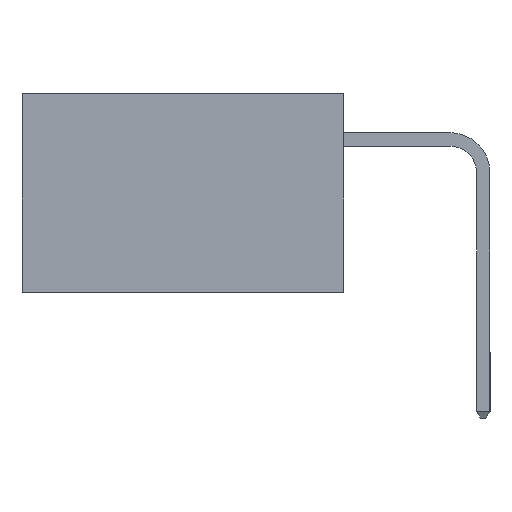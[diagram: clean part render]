
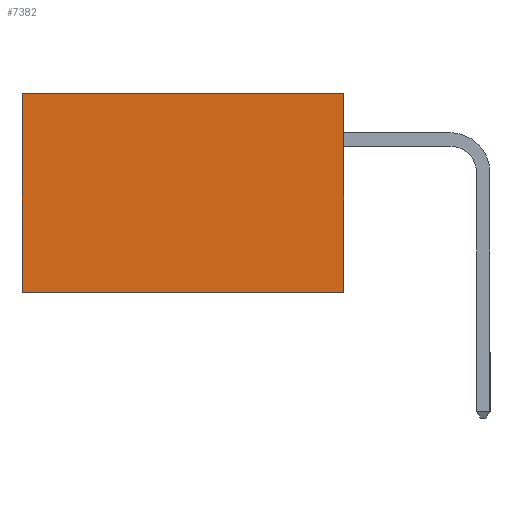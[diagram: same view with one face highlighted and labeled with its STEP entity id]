
A CAD part, left-side view. The second image highlights one B-rep face of the part: STEP entity #7382.
In plain terms, the highlighted planar face has unit normal (-1, 0, 0).
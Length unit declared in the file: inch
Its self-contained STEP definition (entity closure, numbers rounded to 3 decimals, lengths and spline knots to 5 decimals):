
#791 = CARTESIAN_POINT ( 'NONE',  ( 0.298, 0.6, 0. ) ) ;
#913 = VECTOR ( 'NONE', #17034, 39.37008 ) ;
#2879 = DIRECTION ( 'NONE',  ( 0., 1., 0. ) ) ;
#2944 = LINE ( 'NONE', #13796, #9721 ) ;
#3305 = ORIENTED_EDGE ( 'NONE', *, *, #6880, .F. ) ;
#4120 = CARTESIAN_POINT ( 'NONE',  ( 0.298, 0.6, -0.37 ) ) ;
#4395 = EDGE_CURVE ( 'NONE', #13428, #15532, #15515, .T. ) ;
#5298 = CARTESIAN_POINT ( 'NONE',  ( 0.298, 0., -0.37 ) ) ;
#5395 = VERTEX_POINT ( 'NONE', #5298 ) ;
#5860 = LINE ( 'NONE', #5873, #13768 ) ;
#5873 = CARTESIAN_POINT ( 'NONE',  ( 0.298, 0., -0.37 ) ) ;
#5914 = FACE_OUTER_BOUND ( 'NONE', #11638, .T. ) ;
#6100 = DIRECTION ( 'NONE',  ( 0., 0., -1. ) ) ;
#6880 = EDGE_CURVE ( 'NONE', #13428, #5395, #2944, .T. ) ;
#7157 = ORIENTED_EDGE ( 'NONE', *, *, #10382, .T. ) ;
#7382 = ADVANCED_FACE ( 'NONE', ( #5914 ), #11649, .F. ) ;
#7523 = DIRECTION ( 'NONE',  ( 1., 0., 0. ) ) ;
#8343 = LINE ( 'NONE', #17025, #13786 ) ;
#8783 = VERTEX_POINT ( 'NONE', #4120 ) ;
#9721 = VECTOR ( 'NONE', #13739, 39.37008 ) ;
#10382 = EDGE_CURVE ( 'NONE', #15532, #8783, #8343, .T. ) ;
#10694 = AXIS2_PLACEMENT_3D ( 'NONE', #11542, #7523, #15644 ) ;
#11014 = ORIENTED_EDGE ( 'NONE', *, *, #11450, .F. ) ;
#11450 = EDGE_CURVE ( 'NONE', #5395, #8783, #5860, .T. ) ;
#11542 = CARTESIAN_POINT ( 'NONE',  ( 0.298, 0., 0. ) ) ;
#11638 = EDGE_LOOP ( 'NONE', ( #7157, #11014, #3305, #11695 ) ) ;
#11649 = PLANE ( 'NONE',  #10694 ) ;
#11695 = ORIENTED_EDGE ( 'NONE', *, *, #4395, .T. ) ;
#13428 = VERTEX_POINT ( 'NONE', #13780 ) ;
#13739 = DIRECTION ( 'NONE',  ( 0., 0., -1. ) ) ;
#13768 = VECTOR ( 'NONE', #2879, 39.37008 ) ;
#13780 = CARTESIAN_POINT ( 'NONE',  ( 0.298, 0., 0. ) ) ;
#13786 = VECTOR ( 'NONE', #6100, 39.37008 ) ;
#13796 = CARTESIAN_POINT ( 'NONE',  ( 0.298, 0., 0. ) ) ;
#15515 = LINE ( 'NONE', #16462, #913 ) ;
#15532 = VERTEX_POINT ( 'NONE', #791 ) ;
#15644 = DIRECTION ( 'NONE',  ( 0., 0., -1. ) ) ;
#16462 = CARTESIAN_POINT ( 'NONE',  ( 0.298, 0., 0. ) ) ;
#17025 = CARTESIAN_POINT ( 'NONE',  ( 0.298, 0.6, 0. ) ) ;
#17034 = DIRECTION ( 'NONE',  ( 0., 1., 0. ) ) ;
